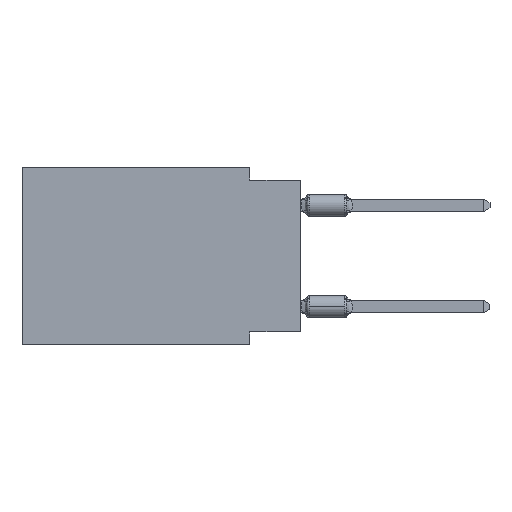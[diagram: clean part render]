
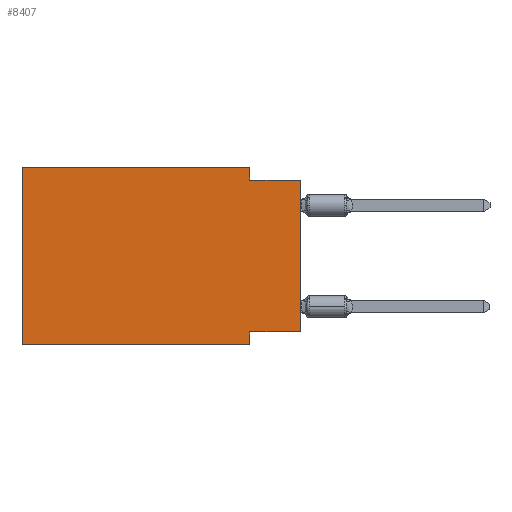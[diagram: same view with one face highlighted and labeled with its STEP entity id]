
A CAD part, left-side view. The second image highlights one B-rep face of the part: STEP entity #8407.
In plain terms, the highlighted planar face has unit normal (-1, 0, 0).
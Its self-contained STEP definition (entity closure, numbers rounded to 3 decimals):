
#709 = EDGE_CURVE ( 'NONE', #9370, #5591, #6640, .T. ) ;
#779 = EDGE_LOOP ( 'NONE', ( #2770, #1178, #7224, #1718, #7561, #3730, #2193, #13446 ) ) ;
#1178 = ORIENTED_EDGE ( 'NONE', *, *, #10395, .F. ) ;
#1333 = CARTESIAN_POINT ( 'NONE',  ( 0., 13.97, -8.89 ) ) ;
#1718 = ORIENTED_EDGE ( 'NONE', *, *, #10217, .F. ) ;
#1774 = VECTOR ( 'NONE', #4349, 1000. ) ;
#1826 = AXIS2_PLACEMENT_3D ( 'NONE', #5390, #8477, #9581 ) ;
#1840 = EDGE_CURVE ( 'NONE', #9370, #3294, #2082, .T. ) ;
#1938 = VECTOR ( 'NONE', #12779, 1000. ) ;
#2051 = CARTESIAN_POINT ( 'NONE',  ( 0., 2.54, -8.89 ) ) ;
#2082 = LINE ( 'NONE', #3252, #9230 ) ;
#2111 = DIRECTION ( 'NONE',  ( 0., 0., -1. ) ) ;
#2154 = CARTESIAN_POINT ( 'NONE',  ( 0., 2.54, -8.255 ) ) ;
#2193 = ORIENTED_EDGE ( 'NONE', *, *, #8012, .F. ) ;
#2570 = VERTEX_POINT ( 'NONE', #7413 ) ;
#2770 = ORIENTED_EDGE ( 'NONE', *, *, #1840, .T. ) ;
#2829 = LINE ( 'NONE', #8133, #10764 ) ;
#2998 = LINE ( 'NONE', #3313, #13526 ) ;
#3252 = CARTESIAN_POINT ( 'NONE',  ( 0., 0., 0. ) ) ;
#3294 = VERTEX_POINT ( 'NONE', #8430 ) ;
#3313 = CARTESIAN_POINT ( 'NONE',  ( 0., 13.97, 0. ) ) ;
#3317 = CARTESIAN_POINT ( 'NONE',  ( 0., 2.54, 0. ) ) ;
#3332 = CARTESIAN_POINT ( 'NONE',  ( 0., 13.97, -8.89 ) ) ;
#3730 = ORIENTED_EDGE ( 'NONE', *, *, #5583, .T. ) ;
#3766 = VECTOR ( 'NONE', #5530, 1000. ) ;
#3799 = VECTOR ( 'NONE', #2111, 1000. ) ;
#4349 = DIRECTION ( 'NONE',  ( 0., 0., -1. ) ) ;
#4415 = LINE ( 'NONE', #3317, #1774 ) ;
#5291 = EDGE_CURVE ( 'NONE', #12707, #5740, #2829, .T. ) ;
#5341 = VERTEX_POINT ( 'NONE', #10534 ) ;
#5390 = CARTESIAN_POINT ( 'NONE',  ( 0., 13.97, 0. ) ) ;
#5530 = DIRECTION ( 'NONE',  ( 0., -1., 0. ) ) ;
#5583 = EDGE_CURVE ( 'NONE', #12707, #2570, #6288, .T. ) ;
#5591 = VERTEX_POINT ( 'NONE', #2154 ) ;
#5740 = VERTEX_POINT ( 'NONE', #7854 ) ;
#5964 = EDGE_CURVE ( 'NONE', #5994, #5341, #4415, .T. ) ;
#5994 = VERTEX_POINT ( 'NONE', #6212 ) ;
#6051 = CARTESIAN_POINT ( 'NONE',  ( 0., 0., -8.255 ) ) ;
#6212 = CARTESIAN_POINT ( 'NONE',  ( 0., 2.54, 0. ) ) ;
#6288 = LINE ( 'NONE', #3332, #3766 ) ;
#6572 = CARTESIAN_POINT ( 'NONE',  ( 0., 0., -8.255 ) ) ;
#6640 = LINE ( 'NONE', #6572, #1938 ) ;
#7018 = DIRECTION ( 'NONE',  ( 0., 0., 1. ) ) ;
#7224 = ORIENTED_EDGE ( 'NONE', *, *, #5964, .F. ) ;
#7305 = DIRECTION ( 'NONE',  ( 0., 0., 1. ) ) ;
#7413 = CARTESIAN_POINT ( 'NONE',  ( 0., 2.54, -8.89 ) ) ;
#7561 = ORIENTED_EDGE ( 'NONE', *, *, #5291, .F. ) ;
#7569 = FACE_OUTER_BOUND ( 'NONE', #779, .T. ) ;
#7854 = CARTESIAN_POINT ( 'NONE',  ( 0., 13.97, 0. ) ) ;
#7908 = LINE ( 'NONE', #9908, #11971 ) ;
#8012 = EDGE_CURVE ( 'NONE', #5591, #2570, #10446, .T. ) ;
#8133 = CARTESIAN_POINT ( 'NONE',  ( 0., 13.97, 0. ) ) ;
#8407 = ADVANCED_FACE ( 'NONE', ( #7569 ), #12742, .F. ) ;
#8430 = CARTESIAN_POINT ( 'NONE',  ( 0., 0., -0.635 ) ) ;
#8477 = DIRECTION ( 'NONE',  ( 1., 0., 0. ) ) ;
#8537 = DIRECTION ( 'NONE',  ( 0., -1., 0. ) ) ;
#9230 = VECTOR ( 'NONE', #7305, 1000. ) ;
#9370 = VERTEX_POINT ( 'NONE', #6051 ) ;
#9581 = DIRECTION ( 'NONE',  ( 0., 0., -1. ) ) ;
#9908 = CARTESIAN_POINT ( 'NONE',  ( 0., 0., -0.635 ) ) ;
#10108 = DIRECTION ( 'NONE',  ( 0., -1., 0. ) ) ;
#10217 = EDGE_CURVE ( 'NONE', #5740, #5994, #2998, .T. ) ;
#10395 = EDGE_CURVE ( 'NONE', #5341, #3294, #7908, .T. ) ;
#10446 = LINE ( 'NONE', #2051, #3799 ) ;
#10534 = CARTESIAN_POINT ( 'NONE',  ( 0., 2.54, -0.635 ) ) ;
#10764 = VECTOR ( 'NONE', #7018, 1000. ) ;
#11971 = VECTOR ( 'NONE', #10108, 1000. ) ;
#12707 = VERTEX_POINT ( 'NONE', #1333 ) ;
#12742 = PLANE ( 'NONE',  #1826 ) ;
#12779 = DIRECTION ( 'NONE',  ( 0., 1., 0. ) ) ;
#13446 = ORIENTED_EDGE ( 'NONE', *, *, #709, .F. ) ;
#13526 = VECTOR ( 'NONE', #8537, 1000. ) ;
